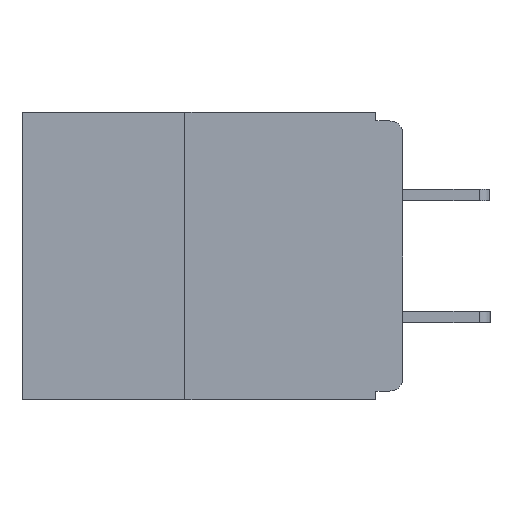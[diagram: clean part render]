
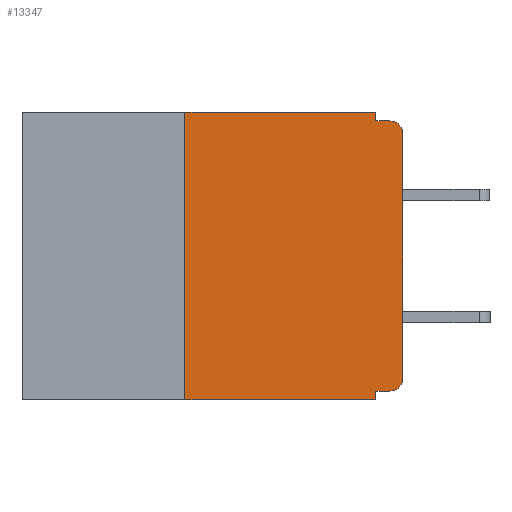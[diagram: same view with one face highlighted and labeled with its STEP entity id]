
A CAD part, left-side view. The second image highlights one B-rep face of the part: STEP entity #13347.
In plain terms, the highlighted planar face has unit normal (-1, 0, 0).
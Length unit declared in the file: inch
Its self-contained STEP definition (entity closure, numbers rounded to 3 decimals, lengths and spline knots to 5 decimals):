
#303 = VECTOR ( 'NONE', #11582, 39.37008 ) ;
#503 = VERTEX_POINT ( 'NONE', #17070 ) ;
#727 = VERTEX_POINT ( 'NONE', #15298 ) ;
#917 = EDGE_CURVE ( 'NONE', #727, #6818, #1861, .T. ) ;
#960 = VECTOR ( 'NONE', #12652, 39.37008 ) ;
#1441 = VECTOR ( 'NONE', #7169, 39.37008 ) ;
#1550 = CIRCLE ( 'NONE', #13682, 0.015 ) ;
#1697 = VECTOR ( 'NONE', #16397, 39.37008 ) ;
#1861 = LINE ( 'NONE', #7055, #1441 ) ;
#1868 = LINE ( 'NONE', #3250, #11960 ) ;
#1983 = CARTESIAN_POINT ( 'NONE',  ( 0., 0.031, -0.01 ) ) ;
#2413 = EDGE_CURVE ( 'NONE', #10287, #503, #13600, .T. ) ;
#2417 = VERTEX_POINT ( 'NONE', #15270 ) ;
#2546 = LINE ( 'NONE', #11083, #1697 ) ;
#2683 = VECTOR ( 'NONE', #15519, 39.37008 ) ;
#2688 = ORIENTED_EDGE ( 'NONE', *, *, #12223, .F. ) ;
#3053 = CARTESIAN_POINT ( 'NONE',  ( 0., 0.031, 0. ) ) ;
#3250 = CARTESIAN_POINT ( 'NONE',  ( 0., 0.437, -0.33 ) ) ;
#3762 = FACE_OUTER_BOUND ( 'NONE', #6236, .T. ) ;
#3953 = AXIS2_PLACEMENT_3D ( 'NONE', #12586, #4336, #13922 ) ;
#3972 = DIRECTION ( 'NONE',  ( 1., 0., 0. ) ) ;
#4044 = VERTEX_POINT ( 'NONE', #15238 ) ;
#4301 = DIRECTION ( 'NONE',  ( 0., 1., 0. ) ) ;
#4336 = DIRECTION ( 'NONE',  ( -1., 0., 0. ) ) ;
#4433 = VECTOR ( 'NONE', #4301, 39.37008 ) ;
#4434 = CARTESIAN_POINT ( 'NONE',  ( 0., 0.25, -0.33 ) ) ;
#4796 = ORIENTED_EDGE ( 'NONE', *, *, #13553, .F. ) ;
#5834 = CARTESIAN_POINT ( 'NONE',  ( 0., 0.015, -0.305 ) ) ;
#6209 = VERTEX_POINT ( 'NONE', #14687 ) ;
#6236 = EDGE_LOOP ( 'NONE', ( #10116, #14110, #15773, #14131, #12295, #10375, #9966, #4796, #2688, #17273 ) ) ;
#6797 = VERTEX_POINT ( 'NONE', #7771 ) ;
#6818 = VERTEX_POINT ( 'NONE', #15921 ) ;
#7055 = CARTESIAN_POINT ( 'NONE',  ( 0., 0.437, 0. ) ) ;
#7169 = DIRECTION ( 'NONE',  ( 0., -1., 0. ) ) ;
#7242 = DIRECTION ( 'NONE',  ( 0., 0., -1. ) ) ;
#7248 = EDGE_CURVE ( 'NONE', #8830, #2417, #1868, .T. ) ;
#7764 = EDGE_CURVE ( 'NONE', #6818, #10287, #15060, .T. ) ;
#7771 = CARTESIAN_POINT ( 'NONE',  ( 0., 0., -0.025 ) ) ;
#8118 = LINE ( 'NONE', #9822, #4433 ) ;
#8830 = VERTEX_POINT ( 'NONE', #4434 ) ;
#9822 = CARTESIAN_POINT ( 'NONE',  ( 0., 0., -0.32 ) ) ;
#9966 = ORIENTED_EDGE ( 'NONE', *, *, #7248, .T. ) ;
#10116 = ORIENTED_EDGE ( 'NONE', *, *, #11903, .T. ) ;
#10194 = CARTESIAN_POINT ( 'NONE',  ( 0., 0.031, -0.33 ) ) ;
#10287 = VERTEX_POINT ( 'NONE', #1983 ) ;
#10375 = ORIENTED_EDGE ( 'NONE', *, *, #12176, .F. ) ;
#10492 = CARTESIAN_POINT ( 'NONE',  ( 0., 0., 0. ) ) ;
#10683 = EDGE_CURVE ( 'NONE', #6209, #13726, #1550, .T. ) ;
#11083 = CARTESIAN_POINT ( 'NONE',  ( 0., 0.25, -0.33 ) ) ;
#11094 = CARTESIAN_POINT ( 'NONE',  ( 0., 0., -0.305 ) ) ;
#11320 = LINE ( 'NONE', #10194, #303 ) ;
#11502 = DIRECTION ( 'NONE',  ( 0., -1., 0. ) ) ;
#11582 = DIRECTION ( 'NONE',  ( 0., 0., -1. ) ) ;
#11872 = DIRECTION ( 'NONE',  ( 0., 0., 1. ) ) ;
#11903 = EDGE_CURVE ( 'NONE', #13726, #6797, #14092, .T. ) ;
#11960 = VECTOR ( 'NONE', #11502, 39.37008 ) ;
#12176 = EDGE_CURVE ( 'NONE', #8830, #727, #2546, .T. ) ;
#12223 = EDGE_CURVE ( 'NONE', #6209, #4044, #8118, .T. ) ;
#12229 = CARTESIAN_POINT ( 'NONE',  ( 0., 0.437, 0. ) ) ;
#12295 = ORIENTED_EDGE ( 'NONE', *, *, #917, .F. ) ;
#12468 = AXIS2_PLACEMENT_3D ( 'NONE', #12229, #3972, #13569 ) ;
#12586 = CARTESIAN_POINT ( 'NONE',  ( 0., 0.015, -0.025 ) ) ;
#12652 = DIRECTION ( 'NONE',  ( 0., 0., -1. ) ) ;
#13347 = ADVANCED_FACE ( 'NONE', ( #3762 ), #17417, .F. ) ;
#13553 = EDGE_CURVE ( 'NONE', #4044, #2417, #11320, .T. ) ;
#13569 = DIRECTION ( 'NONE',  ( 0., 0., -1. ) ) ;
#13600 = LINE ( 'NONE', #15264, #2683 ) ;
#13682 = AXIS2_PLACEMENT_3D ( 'NONE', #5834, #15363, #7242 ) ;
#13695 = VECTOR ( 'NONE', #11872, 39.37008 ) ;
#13726 = VERTEX_POINT ( 'NONE', #11094 ) ;
#13922 = DIRECTION ( 'NONE',  ( 0., 0., -1. ) ) ;
#14092 = LINE ( 'NONE', #10492, #13695 ) ;
#14110 = ORIENTED_EDGE ( 'NONE', *, *, #14917, .T. ) ;
#14131 = ORIENTED_EDGE ( 'NONE', *, *, #7764, .F. ) ;
#14687 = CARTESIAN_POINT ( 'NONE',  ( 0., 0.015, -0.32 ) ) ;
#14917 = EDGE_CURVE ( 'NONE', #6797, #503, #16861, .T. ) ;
#15060 = LINE ( 'NONE', #3053, #960 ) ;
#15238 = CARTESIAN_POINT ( 'NONE',  ( 0., 0.031, -0.32 ) ) ;
#15264 = CARTESIAN_POINT ( 'NONE',  ( 0., 0., -0.01 ) ) ;
#15270 = CARTESIAN_POINT ( 'NONE',  ( 0., 0.031, -0.33 ) ) ;
#15298 = CARTESIAN_POINT ( 'NONE',  ( 0., 0.25, 0. ) ) ;
#15363 = DIRECTION ( 'NONE',  ( -1., 0., 0. ) ) ;
#15519 = DIRECTION ( 'NONE',  ( 0., -1., 0. ) ) ;
#15773 = ORIENTED_EDGE ( 'NONE', *, *, #2413, .F. ) ;
#15921 = CARTESIAN_POINT ( 'NONE',  ( 0., 0.031, 0. ) ) ;
#16397 = DIRECTION ( 'NONE',  ( 0., 0., 1. ) ) ;
#16861 = CIRCLE ( 'NONE', #3953, 0.015 ) ;
#17070 = CARTESIAN_POINT ( 'NONE',  ( 0., 0.015, -0.01 ) ) ;
#17273 = ORIENTED_EDGE ( 'NONE', *, *, #10683, .T. ) ;
#17417 = PLANE ( 'NONE',  #12468 ) ;
